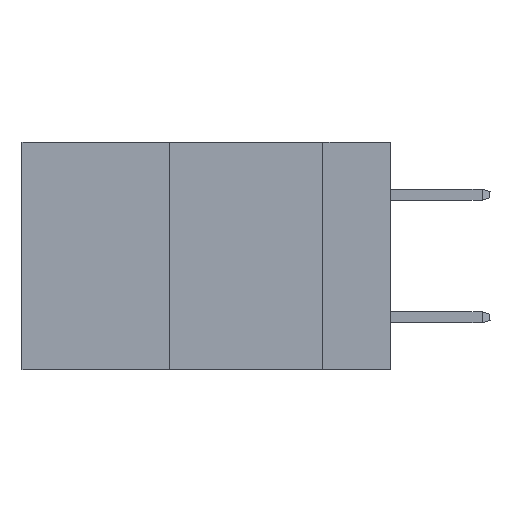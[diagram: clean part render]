
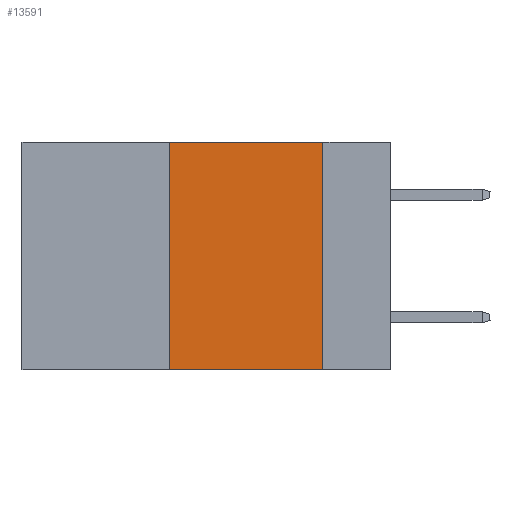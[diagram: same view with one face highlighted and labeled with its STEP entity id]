
A CAD part, left-side view. The second image highlights one B-rep face of the part: STEP entity #13591.
In plain terms, the highlighted planar face has unit normal (-1, 0, 0).
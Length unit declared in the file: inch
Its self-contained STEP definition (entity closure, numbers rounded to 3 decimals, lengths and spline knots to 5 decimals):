
#6 = PLANE ( 'NONE',  #18498 ) ;
#152 = DIRECTION ( 'NONE',  ( 0., 0., -1. ) ) ;
#1309 = LINE ( 'NONE', #11534, #9282 ) ;
#2051 = LINE ( 'NONE', #18709, #8386 ) ;
#2404 = DIRECTION ( 'NONE',  ( 0., -1., 0. ) ) ;
#2962 = EDGE_LOOP ( 'NONE', ( #22095, #6023, #15881, #19741 ) ) ;
#3104 = DIRECTION ( 'NONE',  ( 0., 0., 1. ) ) ;
#3897 = FACE_OUTER_BOUND ( 'NONE', #2962, .T. ) ;
#4529 = EDGE_CURVE ( 'NONE', #12857, #5447, #5133, .T. ) ;
#4865 = VECTOR ( 'NONE', #2404, 39.37008 ) ;
#5133 = LINE ( 'NONE', #6018, #4865 ) ;
#5314 = CARTESIAN_POINT ( 'NONE',  ( 0., 0.6, 0. ) ) ;
#5447 = VERTEX_POINT ( 'NONE', #9058 ) ;
#6018 = CARTESIAN_POINT ( 'NONE',  ( 0., 0.6, 0. ) ) ;
#6023 = ORIENTED_EDGE ( 'NONE', *, *, #4529, .F. ) ;
#6697 = CARTESIAN_POINT ( 'NONE',  ( 0., 0.36, -0.37 ) ) ;
#8386 = VECTOR ( 'NONE', #22119, 39.37008 ) ;
#9058 = CARTESIAN_POINT ( 'NONE',  ( 0., 0.11, 0. ) ) ;
#9282 = VECTOR ( 'NONE', #9689, 39.37008 ) ;
#9689 = DIRECTION ( 'NONE',  ( 0., -1., 0. ) ) ;
#11195 = CARTESIAN_POINT ( 'NONE',  ( 0., 0.11, -0.37 ) ) ;
#11534 = CARTESIAN_POINT ( 'NONE',  ( 0., 0.6, -0.37 ) ) ;
#12191 = EDGE_CURVE ( 'NONE', #5447, #15814, #2051, .T. ) ;
#12857 = VERTEX_POINT ( 'NONE', #13378 ) ;
#12869 = EDGE_CURVE ( 'NONE', #17986, #12857, #22650, .T. ) ;
#13378 = CARTESIAN_POINT ( 'NONE',  ( 0., 0.36, 0. ) ) ;
#13591 = ADVANCED_FACE ( 'NONE', ( #3897 ), #6, .F. ) ;
#15814 = VERTEX_POINT ( 'NONE', #11195 ) ;
#15881 = ORIENTED_EDGE ( 'NONE', *, *, #12869, .F. ) ;
#16127 = DIRECTION ( 'NONE',  ( 1., 0., 0. ) ) ;
#17688 = VECTOR ( 'NONE', #3104, 39.37008 ) ;
#17986 = VERTEX_POINT ( 'NONE', #6697 ) ;
#18498 = AXIS2_PLACEMENT_3D ( 'NONE', #5314, #16127, #152 ) ;
#18709 = CARTESIAN_POINT ( 'NONE',  ( 0., 0.11, 0. ) ) ;
#19741 = ORIENTED_EDGE ( 'NONE', *, *, #22411, .T. ) ;
#22095 = ORIENTED_EDGE ( 'NONE', *, *, #12191, .F. ) ;
#22119 = DIRECTION ( 'NONE',  ( 0., 0., -1. ) ) ;
#22169 = CARTESIAN_POINT ( 'NONE',  ( 0., 0.36, 0. ) ) ;
#22411 = EDGE_CURVE ( 'NONE', #17986, #15814, #1309, .T. ) ;
#22650 = LINE ( 'NONE', #22169, #17688 ) ;
